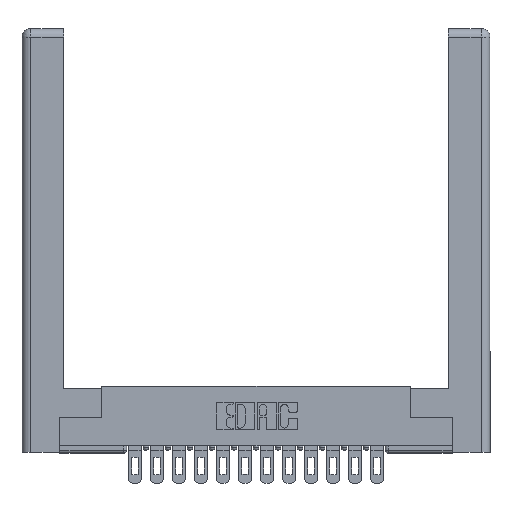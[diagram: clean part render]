
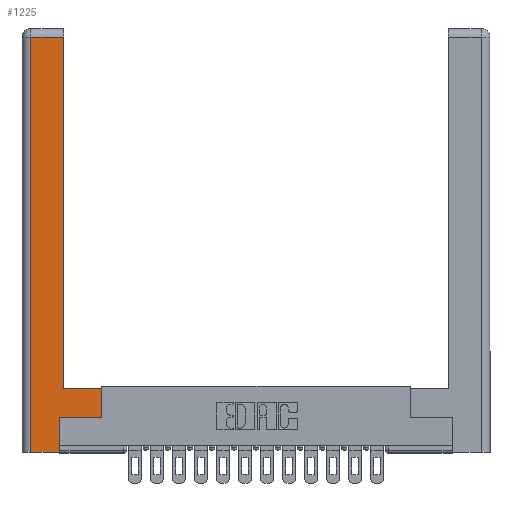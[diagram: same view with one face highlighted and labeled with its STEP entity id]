
A CAD part, top view. The second image highlights one B-rep face of the part: STEP entity #1225.
In plain terms, the highlighted planar face has unit normal (0, 0, 1).
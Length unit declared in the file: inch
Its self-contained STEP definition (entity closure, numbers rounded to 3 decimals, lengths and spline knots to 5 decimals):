
#65 = ORIENTED_EDGE ( 'NONE', *, *, #7788, .T. ) ;
#89 = VERTEX_POINT ( 'NONE', #16111 ) ;
#519 = CARTESIAN_POINT ( 'NONE',  ( 0.565, 0.45, 0. ) ) ;
#1220 = ORIENTED_EDGE ( 'NONE', *, *, #14829, .T. ) ;
#1225 = ADVANCED_FACE ( 'NONE', ( #8852 ), #8206, .F. ) ;
#1289 = VERTEX_POINT ( 'NONE', #6278 ) ;
#2287 = VECTOR ( 'NONE', #5707, 39.37008 ) ;
#2750 = LINE ( 'NONE', #14284, #16606 ) ;
#3114 = DIRECTION ( 'NONE',  ( -1., 0., 0. ) ) ;
#3281 = VECTOR ( 'NONE', #14298, 39.37008 ) ;
#4048 = VECTOR ( 'NONE', #3114, 39.37008 ) ;
#4214 = DIRECTION ( 'NONE',  ( 0., 0., -1. ) ) ;
#4228 = ORIENTED_EDGE ( 'NONE', *, *, #8495, .T. ) ;
#4256 = VERTEX_POINT ( 'NONE', #14263 ) ;
#4346 = CARTESIAN_POINT ( 'NONE',  ( 0.265, 0., 0. ) ) ;
#4412 = LINE ( 'NONE', #10510, #15739 ) ;
#4654 = DIRECTION ( 'NONE',  ( 0., 1., 0. ) ) ;
#4830 = EDGE_CURVE ( 'NONE', #7234, #9658, #10438, .T. ) ;
#5304 = LINE ( 'NONE', #9724, #4048 ) ;
#5319 = VERTEX_POINT ( 'NONE', #14164 ) ;
#5447 = LINE ( 'NONE', #16770, #8392 ) ;
#5576 = CARTESIAN_POINT ( 'NONE',  ( 0., 0., 0. ) ) ;
#5707 = DIRECTION ( 'NONE',  ( 1., 0., 0. ) ) ;
#5983 = AXIS2_PLACEMENT_3D ( 'NONE', #5576, #4214, #14882 ) ;
#6197 = VERTEX_POINT ( 'NONE', #16004 ) ;
#6278 = CARTESIAN_POINT ( 'NONE',  ( 0.265, 0.245, 0. ) ) ;
#6680 = EDGE_CURVE ( 'NONE', #4256, #6197, #2750, .T. ) ;
#7137 = VECTOR ( 'NONE', #4654, 39.37008 ) ;
#7234 = VERTEX_POINT ( 'NONE', #7262 ) ;
#7262 = CARTESIAN_POINT ( 'NONE',  ( 0.295, 0.45, 0. ) ) ;
#7714 = EDGE_CURVE ( 'NONE', #6197, #5319, #11130, .T. ) ;
#7788 = EDGE_CURVE ( 'NONE', #5319, #1289, #17401, .T. ) ;
#8206 = PLANE ( 'NONE',  #5983 ) ;
#8392 = VECTOR ( 'NONE', #12860, 39.37008 ) ;
#8415 = CARTESIAN_POINT ( 'NONE',  ( 0.565, 0.245, 0. ) ) ;
#8495 = EDGE_CURVE ( 'NONE', #1289, #13866, #5447, .T. ) ;
#8637 = DIRECTION ( 'NONE',  ( 0., 1., 0. ) ) ;
#8852 = FACE_OUTER_BOUND ( 'NONE', #16254, .T. ) ;
#9014 = DIRECTION ( 'NONE',  ( 0., -1., 0. ) ) ;
#9658 = VERTEX_POINT ( 'NONE', #9794 ) ;
#9724 = CARTESIAN_POINT ( 'NONE',  ( 0.295, 0.45, 0. ) ) ;
#9794 = CARTESIAN_POINT ( 'NONE',  ( 0.295, 2.94, 0. ) ) ;
#10438 = LINE ( 'NONE', #14080, #3281 ) ;
#10510 = CARTESIAN_POINT ( 'NONE',  ( 0.0615, 2.94, 0. ) ) ;
#10894 = EDGE_CURVE ( 'NONE', #13866, #89, #13349, .T. ) ;
#11130 = LINE ( 'NONE', #4346, #2287 ) ;
#12500 = ORIENTED_EDGE ( 'NONE', *, *, #13457, .T. ) ;
#12860 = DIRECTION ( 'NONE',  ( 1., 0., 0. ) ) ;
#13349 = LINE ( 'NONE', #519, #13757 ) ;
#13378 = ORIENTED_EDGE ( 'NONE', *, *, #4830, .T. ) ;
#13457 = EDGE_CURVE ( 'NONE', #89, #7234, #5304, .T. ) ;
#13757 = VECTOR ( 'NONE', #8637, 39.37008 ) ;
#13866 = VERTEX_POINT ( 'NONE', #8415 ) ;
#13922 = ORIENTED_EDGE ( 'NONE', *, *, #7714, .T. ) ;
#14080 = CARTESIAN_POINT ( 'NONE',  ( 0.295, 3., 0. ) ) ;
#14164 = CARTESIAN_POINT ( 'NONE',  ( 0.265, 0., 0. ) ) ;
#14263 = CARTESIAN_POINT ( 'NONE',  ( 0.0615, 2.94, 0. ) ) ;
#14284 = CARTESIAN_POINT ( 'NONE',  ( 0.0615, 0., 0. ) ) ;
#14298 = DIRECTION ( 'NONE',  ( 0., 1., 0. ) ) ;
#14829 = EDGE_CURVE ( 'NONE', #9658, #4256, #4412, .T. ) ;
#14882 = DIRECTION ( 'NONE',  ( -1., 0., 0. ) ) ;
#15131 = ORIENTED_EDGE ( 'NONE', *, *, #6680, .T. ) ;
#15441 = CARTESIAN_POINT ( 'NONE',  ( 0.265, 0.245, 0. ) ) ;
#15739 = VECTOR ( 'NONE', #17404, 39.37008 ) ;
#16004 = CARTESIAN_POINT ( 'NONE',  ( 0.0615, 0., 0. ) ) ;
#16111 = CARTESIAN_POINT ( 'NONE',  ( 0.565, 0.45, 0. ) ) ;
#16254 = EDGE_LOOP ( 'NONE', ( #13378, #1220, #15131, #13922, #65, #4228, #17335, #12500 ) ) ;
#16606 = VECTOR ( 'NONE', #9014, 39.37008 ) ;
#16770 = CARTESIAN_POINT ( 'NONE',  ( 0.565, 0.245, 0. ) ) ;
#17335 = ORIENTED_EDGE ( 'NONE', *, *, #10894, .T. ) ;
#17401 = LINE ( 'NONE', #15441, #7137 ) ;
#17404 = DIRECTION ( 'NONE',  ( -1., 0., 0. ) ) ;
